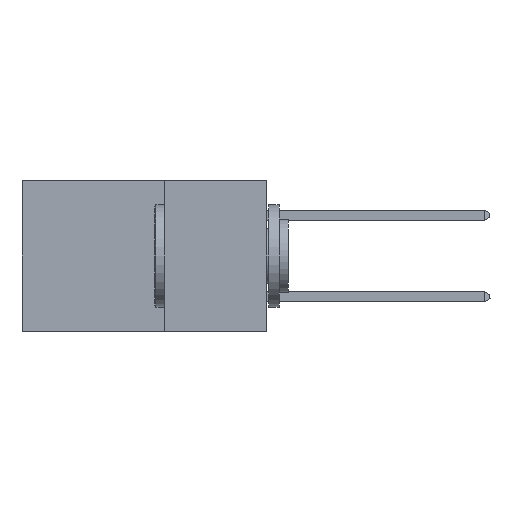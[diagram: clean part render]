
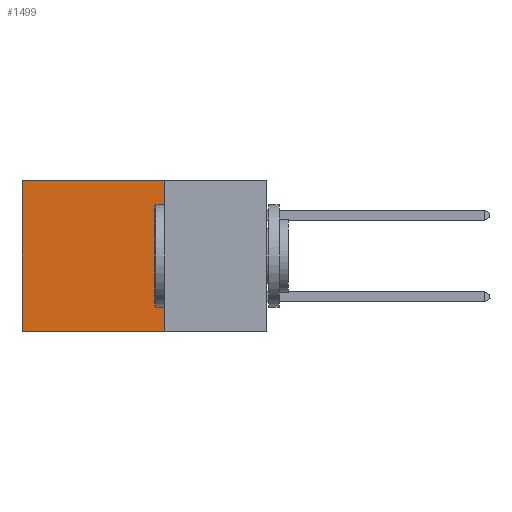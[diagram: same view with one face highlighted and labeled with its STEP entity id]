
A CAD part, left-side view. The second image highlights one B-rep face of the part: STEP entity #1499.
In plain terms, the highlighted planar face has unit normal (-1, 0, 0).
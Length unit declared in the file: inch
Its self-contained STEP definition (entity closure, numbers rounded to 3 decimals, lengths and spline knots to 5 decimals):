
#109 = LINE ( 'NONE', #13031, #9564 ) ;
#269 = VECTOR ( 'NONE', #6978, 39.37008 ) ;
#416 = DIRECTION ( 'NONE',  ( 0., 0., -1. ) ) ;
#494 = VERTEX_POINT ( 'NONE', #15226 ) ;
#649 = CARTESIAN_POINT ( 'NONE',  ( 0.2875, 0.25, 0. ) ) ;
#892 = VERTEX_POINT ( 'NONE', #5349 ) ;
#938 = CARTESIAN_POINT ( 'NONE',  ( 0.2875, 0.6, -0.37 ) ) ;
#1499 = ADVANCED_FACE ( 'NONE', ( #7930 ), #13494, .F. ) ;
#1795 = DIRECTION ( 'NONE',  ( 0., 0., -1. ) ) ;
#2060 = EDGE_CURVE ( 'NONE', #892, #494, #15997, .T. ) ;
#5217 = DIRECTION ( 'NONE',  ( 0., 1., 0. ) ) ;
#5349 = CARTESIAN_POINT ( 'NONE',  ( 0.2875, 0.25, 0. ) ) ;
#5451 = VERTEX_POINT ( 'NONE', #7906 ) ;
#5765 = DIRECTION ( 'NONE',  ( 1., 0., 0. ) ) ;
#6978 = DIRECTION ( 'NONE',  ( 0., 1., 0. ) ) ;
#7677 = CARTESIAN_POINT ( 'NONE',  ( 0.2875, 0.25, 0. ) ) ;
#7830 = DIRECTION ( 'NONE',  ( 0., 0., -1. ) ) ;
#7906 = CARTESIAN_POINT ( 'NONE',  ( 0.2875, 0.6, 0. ) ) ;
#7930 = FACE_OUTER_BOUND ( 'NONE', #14944, .T. ) ;
#8638 = AXIS2_PLACEMENT_3D ( 'NONE', #649, #5765, #1795 ) ;
#9149 = ORIENTED_EDGE ( 'NONE', *, *, #14508, .T. ) ;
#9313 = LINE ( 'NONE', #14792, #269 ) ;
#9564 = VECTOR ( 'NONE', #7830, 39.37008 ) ;
#10278 = EDGE_CURVE ( 'NONE', #494, #11995, #9313, .T. ) ;
#11248 = ORIENTED_EDGE ( 'NONE', *, *, #2060, .F. ) ;
#11515 = VECTOR ( 'NONE', #416, 39.37008 ) ;
#11995 = VERTEX_POINT ( 'NONE', #938 ) ;
#12097 = ORIENTED_EDGE ( 'NONE', *, *, #12214, .T. ) ;
#12214 = EDGE_CURVE ( 'NONE', #892, #5451, #13724, .T. ) ;
#12502 = VECTOR ( 'NONE', #5217, 39.37008 ) ;
#12726 = ORIENTED_EDGE ( 'NONE', *, *, #10278, .F. ) ;
#13031 = CARTESIAN_POINT ( 'NONE',  ( 0.2875, 0.6, 0. ) ) ;
#13494 = PLANE ( 'NONE',  #8638 ) ;
#13724 = LINE ( 'NONE', #15455, #12502 ) ;
#14508 = EDGE_CURVE ( 'NONE', #5451, #11995, #109, .T. ) ;
#14792 = CARTESIAN_POINT ( 'NONE',  ( 0.2875, 0.25, -0.37 ) ) ;
#14944 = EDGE_LOOP ( 'NONE', ( #9149, #12726, #11248, #12097 ) ) ;
#15226 = CARTESIAN_POINT ( 'NONE',  ( 0.2875, 0.25, -0.37 ) ) ;
#15455 = CARTESIAN_POINT ( 'NONE',  ( 0.2875, 0.25, 0. ) ) ;
#15997 = LINE ( 'NONE', #7677, #11515 ) ;
